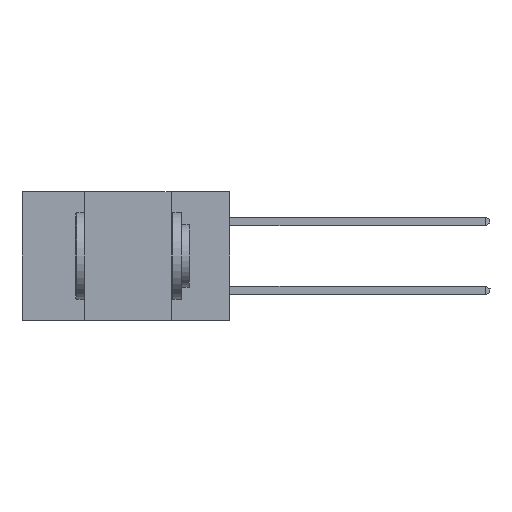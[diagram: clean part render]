
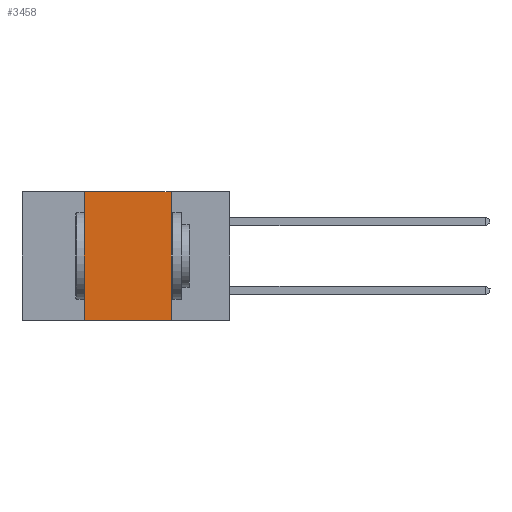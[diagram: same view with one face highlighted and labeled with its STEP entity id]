
A CAD part, left-side view. The second image highlights one B-rep face of the part: STEP entity #3458.
In plain terms, the highlighted planar face has unit normal (-1, 0, 0).
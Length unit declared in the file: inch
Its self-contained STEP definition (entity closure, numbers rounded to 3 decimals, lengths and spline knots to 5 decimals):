
#31 = VERTEX_POINT ( 'NONE', #720 ) ;
#720 = CARTESIAN_POINT ( 'NONE',  ( 0., 0.42, -0.37 ) ) ;
#903 = ORIENTED_EDGE ( 'NONE', *, *, #28471, .F. ) ;
#3458 = ADVANCED_FACE ( 'NONE', ( #22943 ), #13325, .F. ) ;
#3928 = EDGE_CURVE ( 'NONE', #4623, #27696, #12511, .T. ) ;
#4219 = VECTOR ( 'NONE', #26849, 39.37008 ) ;
#4329 = CARTESIAN_POINT ( 'NONE',  ( 0., 0.17, 0. ) ) ;
#4581 = CARTESIAN_POINT ( 'NONE',  ( 0., 0.6, 0. ) ) ;
#4623 = VERTEX_POINT ( 'NONE', #4329 ) ;
#5041 = DIRECTION ( 'NONE',  ( 0., -1., 0. ) ) ;
#8971 = DIRECTION ( 'NONE',  ( 1., 0., 0. ) ) ;
#9028 = LINE ( 'NONE', #11366, #4219 ) ;
#10220 = EDGE_LOOP ( 'NONE', ( #11242, #13488, #903, #14155 ) ) ;
#11242 = ORIENTED_EDGE ( 'NONE', *, *, #3928, .F. ) ;
#11366 = CARTESIAN_POINT ( 'NONE',  ( 0., 0.42, 0. ) ) ;
#12511 = LINE ( 'NONE', #19378, #17733 ) ;
#13325 = PLANE ( 'NONE',  #22429 ) ;
#13488 = ORIENTED_EDGE ( 'NONE', *, *, #21075, .F. ) ;
#14155 = ORIENTED_EDGE ( 'NONE', *, *, #15292, .T. ) ;
#15117 = LINE ( 'NONE', #4581, #19940 ) ;
#15292 = EDGE_CURVE ( 'NONE', #31, #27696, #28055, .T. ) ;
#15460 = CARTESIAN_POINT ( 'NONE',  ( 0., 0.17, -0.37 ) ) ;
#15542 = DIRECTION ( 'NONE',  ( 0., 0., -1. ) ) ;
#16279 = VECTOR ( 'NONE', #5041, 39.37008 ) ;
#17733 = VECTOR ( 'NONE', #28162, 39.37008 ) ;
#17740 = DIRECTION ( 'NONE',  ( 0., -1., 0. ) ) ;
#19157 = CARTESIAN_POINT ( 'NONE',  ( 0., 0.42, 0. ) ) ;
#19378 = CARTESIAN_POINT ( 'NONE',  ( 0., 0.17, 0. ) ) ;
#19940 = VECTOR ( 'NONE', #17740, 39.37008 ) ;
#20319 = CARTESIAN_POINT ( 'NONE',  ( 0., 0.6, -0.37 ) ) ;
#21075 = EDGE_CURVE ( 'NONE', #25351, #4623, #15117, .T. ) ;
#22429 = AXIS2_PLACEMENT_3D ( 'NONE', #26683, #8971, #15542 ) ;
#22943 = FACE_OUTER_BOUND ( 'NONE', #10220, .T. ) ;
#25351 = VERTEX_POINT ( 'NONE', #19157 ) ;
#26683 = CARTESIAN_POINT ( 'NONE',  ( 0., 0.6, 0. ) ) ;
#26849 = DIRECTION ( 'NONE',  ( 0., 0., 1. ) ) ;
#27696 = VERTEX_POINT ( 'NONE', #15460 ) ;
#28055 = LINE ( 'NONE', #20319, #16279 ) ;
#28162 = DIRECTION ( 'NONE',  ( 0., 0., -1. ) ) ;
#28471 = EDGE_CURVE ( 'NONE', #31, #25351, #9028, .T. ) ;
